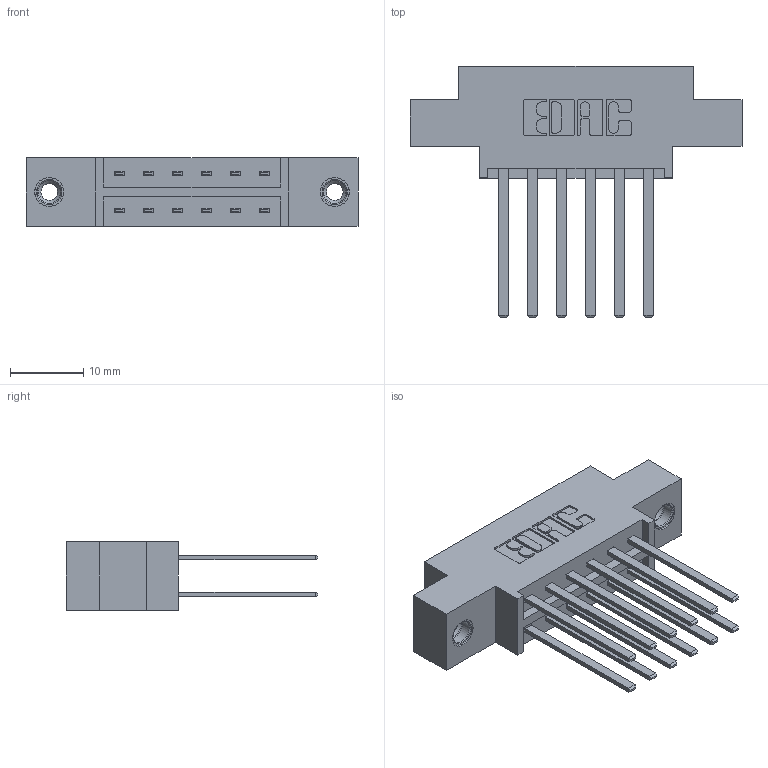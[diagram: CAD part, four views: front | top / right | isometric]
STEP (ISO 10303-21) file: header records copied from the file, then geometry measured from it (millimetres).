
FILE_DESCRIPTION (( 'STEP AP203' ), '1' );
FILE_NAME ('833-012-544-808.STEP', '2020-05-30T22:30:56', ( '' ), ( '' ), 'SwSTEP 2.0', 'SolidWorks 2020', '' );
FILE_SCHEMA (( 'CONFIG_CONTROL_DESIGN' ));
Length unit declared in the file: inch
Products named in the file (4): 833-012-544-808; 345-250-001_345-250-003-102; 833 Part_Offset - .156 Dia - TI; 345-292-001_345-293-144
Assembly tree (15 placements, depth 2):
  833-012-544-808
    833 Part_Offset - .156 Dia - TI
    345-292-001_345-293-144  x12
    345-250-001_345-250-003-102  x2
Bounding box: 45.31 x 34.3 x 9.4 mm (x, y, z)
Volume: 4223.5 mm3; surface area: 5390.6 mm2
Topology: 15 solids, 15 shells, 730 faces, 2103 edges, 1378 vertices
Faces by surface type: plane 490, cylinder 224, cone 12, torus 4
Entity records: 9650 total; most frequent: CARTESIAN_POINT 1625, ORIENTED_EDGE 1554, DIRECTION 1479, EDGE_CURVE 777, VECTOR 633, LINE 633, VERTEX_POINT 512, AXIS2_PLACEMENT_3D 423
